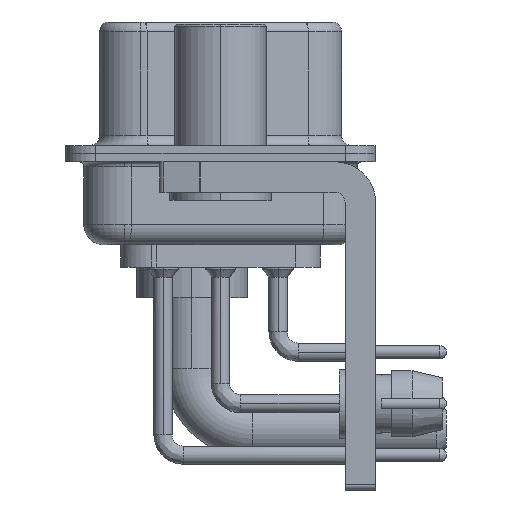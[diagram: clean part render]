
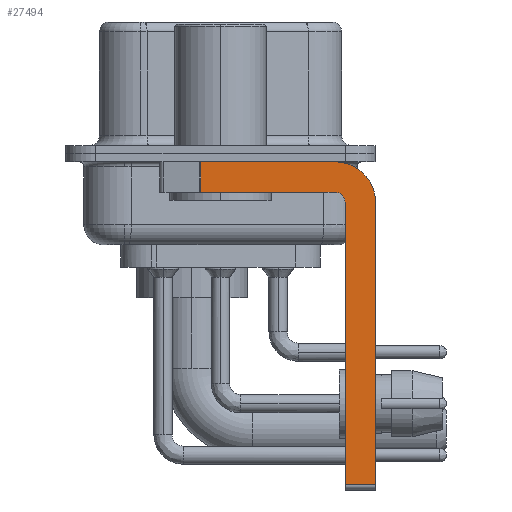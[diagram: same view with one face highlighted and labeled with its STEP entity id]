
A CAD part, left-side view. The second image highlights one B-rep face of the part: STEP entity #27494.
In plain terms, the highlighted planar face has unit normal (-1, 0, 0).
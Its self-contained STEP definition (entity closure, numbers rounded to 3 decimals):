
#297 = LINE ( 'NONE', #24855, #37135 ) ;
#597 = ORIENTED_EDGE ( 'NONE', *, *, #39545, .F. ) ;
#1729 = VECTOR ( 'NONE', #23990, 1000. ) ;
#2014 = PLANE ( 'NONE',  #28739 ) ;
#2043 = AXIS2_PLACEMENT_3D ( 'NONE', #35643, #7700, #10528 ) ;
#3625 = CARTESIAN_POINT ( 'NONE',  ( -2.9, -5.65, -2.4 ) ) ;
#3990 = CIRCLE ( 'NONE', #2043, 0.5 ) ;
#4230 = VECTOR ( 'NONE', #6034, 1000. ) ;
#4867 = VERTEX_POINT ( 'NONE', #21226 ) ;
#5465 = EDGE_CURVE ( 'NONE', #30185, #4867, #14732, .T. ) ;
#5488 = VECTOR ( 'NONE', #38404, 1000. ) ;
#6034 = DIRECTION ( 'NONE',  ( 0., 0., 1. ) ) ;
#7004 = VERTEX_POINT ( 'NONE', #25979 ) ;
#7214 = AXIS2_PLACEMENT_3D ( 'NONE', #34681, #22400, #22591 ) ;
#7700 = DIRECTION ( 'NONE',  ( -1., 0., 0. ) ) ;
#7766 = CARTESIAN_POINT ( 'NONE',  ( -2.9, -7.65, -16.35 ) ) ;
#7769 = ORIENTED_EDGE ( 'NONE', *, *, #5465, .T. ) ;
#8321 = CARTESIAN_POINT ( 'NONE',  ( -2.9, 0.978, -1.9 ) ) ;
#9634 = EDGE_CURVE ( 'NONE', #38176, #4867, #26122, .T. ) ;
#9848 = EDGE_CURVE ( 'NONE', #30185, #31653, #34560, .T. ) ;
#9938 = VECTOR ( 'NONE', #34157, 1000. ) ;
#10181 = LINE ( 'NONE', #15392, #16566 ) ;
#10528 = DIRECTION ( 'NONE',  ( 0., 0., 1. ) ) ;
#14338 = ORIENTED_EDGE ( 'NONE', *, *, #28072, .F. ) ;
#14732 = LINE ( 'NONE', #8321, #1729 ) ;
#15061 = LINE ( 'NONE', #36599, #4230 ) ;
#15331 = VERTEX_POINT ( 'NONE', #7766 ) ;
#15392 = CARTESIAN_POINT ( 'NONE',  ( -2.9, -7.65, -2.4 ) ) ;
#15927 = DIRECTION ( 'NONE',  ( 1., 0., 0. ) ) ;
#16566 = VECTOR ( 'NONE', #31096, 1000. ) ;
#18500 = DIRECTION ( 'NONE',  ( 0., 0., -1. ) ) ;
#20267 = ORIENTED_EDGE ( 'NONE', *, *, #9848, .F. ) ;
#20295 = CARTESIAN_POINT ( 'NONE',  ( -2.9, -5.65, -1.9 ) ) ;
#20799 = EDGE_CURVE ( 'NONE', #31653, #25526, #29651, .T. ) ;
#21212 = CARTESIAN_POINT ( 'NONE',  ( -2.9, 0.978, -0.4 ) ) ;
#21226 = CARTESIAN_POINT ( 'NONE',  ( -2.9, 0.978, -1.9 ) ) ;
#22135 = ORIENTED_EDGE ( 'NONE', *, *, #20799, .F. ) ;
#22400 = DIRECTION ( 'NONE',  ( 1., 0., 0. ) ) ;
#22591 = DIRECTION ( 'NONE',  ( 0., 0., -1. ) ) ;
#23990 = DIRECTION ( 'NONE',  ( 0., 0., -1. ) ) ;
#24208 = EDGE_CURVE ( 'NONE', #7004, #32808, #15061, .T. ) ;
#24408 = ORIENTED_EDGE ( 'NONE', *, *, #9634, .F. ) ;
#24855 = CARTESIAN_POINT ( 'NONE',  ( -2.9, -5.65, -16.35 ) ) ;
#25526 = VERTEX_POINT ( 'NONE', #36118 ) ;
#25597 = EDGE_LOOP ( 'NONE', ( #20267, #7769, #24408, #597, #34664, #28851, #14338, #22135 ) ) ;
#25979 = CARTESIAN_POINT ( 'NONE',  ( -2.9, -6.15, -16.35 ) ) ;
#26122 = LINE ( 'NONE', #35397, #5488 ) ;
#27494 = ADVANCED_FACE ( 'NONE', ( #29576 ), #2014, .F. ) ;
#28072 = EDGE_CURVE ( 'NONE', #25526, #15331, #10181, .T. ) ;
#28123 = EDGE_CURVE ( 'NONE', #7004, #15331, #297, .T. ) ;
#28739 = AXIS2_PLACEMENT_3D ( 'NONE', #3625, #15927, #18500 ) ;
#28851 = ORIENTED_EDGE ( 'NONE', *, *, #28123, .T. ) ;
#29576 = FACE_OUTER_BOUND ( 'NONE', #25597, .T. ) ;
#29651 = CIRCLE ( 'NONE', #7214, 2. ) ;
#30185 = VERTEX_POINT ( 'NONE', #21212 ) ;
#31096 = DIRECTION ( 'NONE',  ( 0., 0., -1. ) ) ;
#31653 = VERTEX_POINT ( 'NONE', #38103 ) ;
#32808 = VERTEX_POINT ( 'NONE', #35371 ) ;
#34157 = DIRECTION ( 'NONE',  ( 0., -1., 0. ) ) ;
#34560 = LINE ( 'NONE', #34958, #9938 ) ;
#34664 = ORIENTED_EDGE ( 'NONE', *, *, #24208, .F. ) ;
#34681 = CARTESIAN_POINT ( 'NONE',  ( -2.9, -5.65, -2.4 ) ) ;
#34958 = CARTESIAN_POINT ( 'NONE',  ( -2.9, 3., -0.4 ) ) ;
#35371 = CARTESIAN_POINT ( 'NONE',  ( -2.9, -6.15, -2.4 ) ) ;
#35397 = CARTESIAN_POINT ( 'NONE',  ( -2.9, -5.65, -1.9 ) ) ;
#35643 = CARTESIAN_POINT ( 'NONE',  ( -2.9, -5.65, -2.4 ) ) ;
#36118 = CARTESIAN_POINT ( 'NONE',  ( -2.9, -7.65, -2.4 ) ) ;
#36599 = CARTESIAN_POINT ( 'NONE',  ( -2.9, -6.15, -16.6 ) ) ;
#37128 = DIRECTION ( 'NONE',  ( 0., -1., 0. ) ) ;
#37135 = VECTOR ( 'NONE', #37128, 1000. ) ;
#38103 = CARTESIAN_POINT ( 'NONE',  ( -2.9, -5.65, -0.4 ) ) ;
#38176 = VERTEX_POINT ( 'NONE', #20295 ) ;
#38404 = DIRECTION ( 'NONE',  ( 0., 1., 0. ) ) ;
#39545 = EDGE_CURVE ( 'NONE', #32808, #38176, #3990, .T. ) ;
